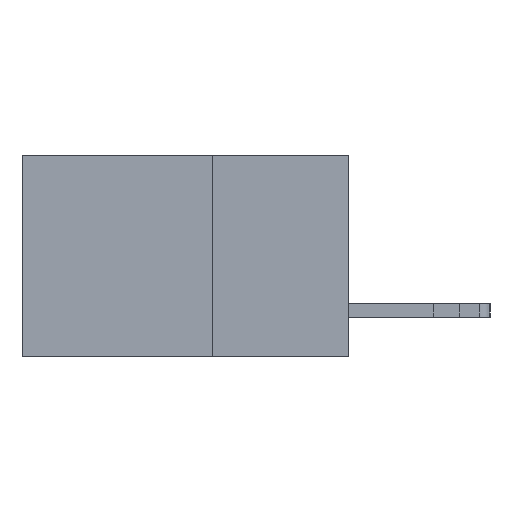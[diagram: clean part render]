
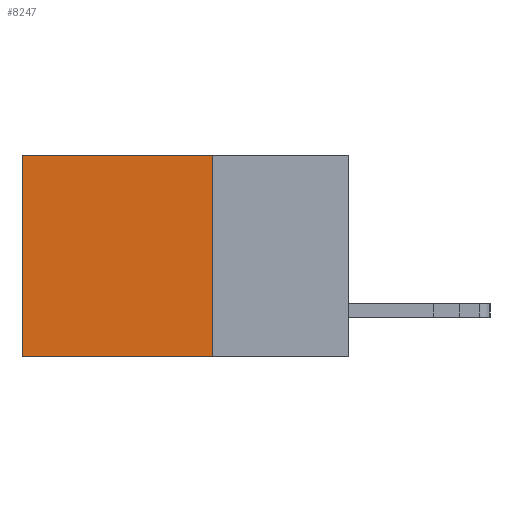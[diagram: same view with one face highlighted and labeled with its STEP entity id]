
A CAD part, left-side view. The second image highlights one B-rep face of the part: STEP entity #8247.
In plain terms, the highlighted planar face has unit normal (-1, 0, 0).
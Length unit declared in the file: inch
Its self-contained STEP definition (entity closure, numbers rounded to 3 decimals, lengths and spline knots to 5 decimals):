
#58 = LINE ( 'NONE', #1725, #9372 ) ;
#196 = EDGE_CURVE ( 'NONE', #7081, #7991, #9831, .T. ) ;
#206 = CARTESIAN_POINT ( 'NONE',  ( 0.2615, 0.6, -0.37 ) ) ;
#398 = CARTESIAN_POINT ( 'NONE',  ( 0.2615, 0.6, 0. ) ) ;
#737 = CARTESIAN_POINT ( 'NONE',  ( 0.2615, 0.6, -0.37 ) ) ;
#1038 = CARTESIAN_POINT ( 'NONE',  ( 0.2615, 0.25, -0.37 ) ) ;
#1725 = CARTESIAN_POINT ( 'NONE',  ( 0.2615, 0.25, 0. ) ) ;
#2247 = VERTEX_POINT ( 'NONE', #10258 ) ;
#2459 = CARTESIAN_POINT ( 'NONE',  ( 0.2615, 0.25, -0.37 ) ) ;
#2543 = LINE ( 'NONE', #10056, #9605 ) ;
#2704 = DIRECTION ( 'NONE',  ( 0., 1., 0. ) ) ;
#3026 = EDGE_LOOP ( 'NONE', ( #6191, #3758, #5451, #11127 ) ) ;
#3758 = ORIENTED_EDGE ( 'NONE', *, *, #8697, .F. ) ;
#3818 = AXIS2_PLACEMENT_3D ( 'NONE', #9420, #4006, #10287 ) ;
#4006 = DIRECTION ( 'NONE',  ( 1., 0., 0. ) ) ;
#4918 = LINE ( 'NONE', #1038, #11687 ) ;
#5451 = ORIENTED_EDGE ( 'NONE', *, *, #6013, .F. ) ;
#6013 = EDGE_CURVE ( 'NONE', #2247, #9161, #4918, .T. ) ;
#6191 = ORIENTED_EDGE ( 'NONE', *, *, #196, .T. ) ;
#6464 = EDGE_CURVE ( 'NONE', #2247, #7081, #58, .T. ) ;
#7081 = VERTEX_POINT ( 'NONE', #398 ) ;
#7581 = DIRECTION ( 'NONE',  ( 0., 0., -1. ) ) ;
#7668 = PLANE ( 'NONE',  #3818 ) ;
#7862 = FACE_OUTER_BOUND ( 'NONE', #3026, .T. ) ;
#7991 = VERTEX_POINT ( 'NONE', #737 ) ;
#8247 = ADVANCED_FACE ( 'NONE', ( #7862 ), #7668, .F. ) ;
#8697 = EDGE_CURVE ( 'NONE', #9161, #7991, #2543, .T. ) ;
#9161 = VERTEX_POINT ( 'NONE', #2459 ) ;
#9372 = VECTOR ( 'NONE', #2704, 39.37008 ) ;
#9406 = DIRECTION ( 'NONE',  ( 0., 0., -1. ) ) ;
#9420 = CARTESIAN_POINT ( 'NONE',  ( 0.2615, 0.25, -0.37 ) ) ;
#9556 = VECTOR ( 'NONE', #7581, 39.37008 ) ;
#9605 = VECTOR ( 'NONE', #11787, 39.37008 ) ;
#9831 = LINE ( 'NONE', #206, #9556 ) ;
#10056 = CARTESIAN_POINT ( 'NONE',  ( 0.2615, 0.25, -0.37 ) ) ;
#10258 = CARTESIAN_POINT ( 'NONE',  ( 0.2615, 0.25, 0. ) ) ;
#10287 = DIRECTION ( 'NONE',  ( 0., 0., -1. ) ) ;
#11127 = ORIENTED_EDGE ( 'NONE', *, *, #6464, .T. ) ;
#11687 = VECTOR ( 'NONE', #9406, 39.37008 ) ;
#11787 = DIRECTION ( 'NONE',  ( 0., 1., 0. ) ) ;
